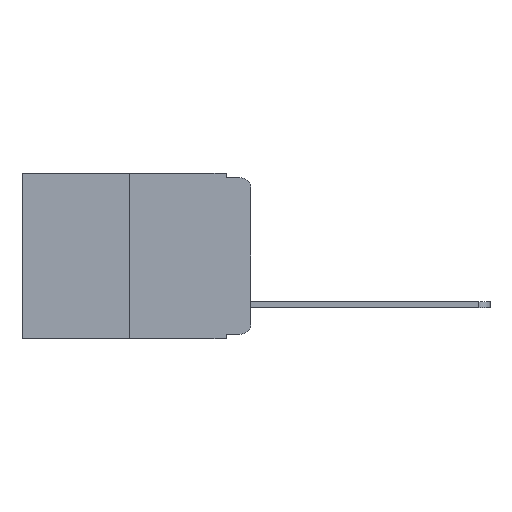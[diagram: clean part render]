
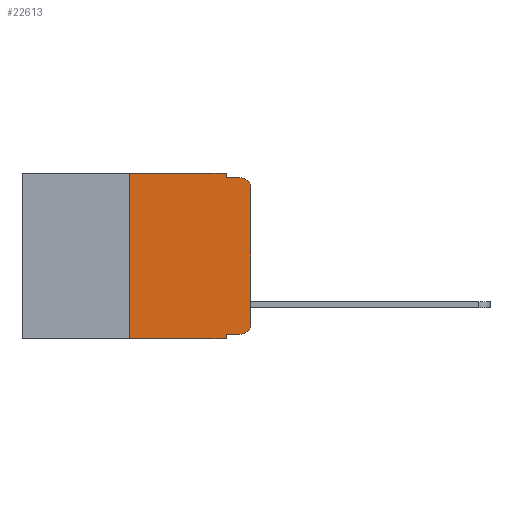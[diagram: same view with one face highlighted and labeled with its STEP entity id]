
A CAD part, left-side view. The second image highlights one B-rep face of the part: STEP entity #22613.
In plain terms, the highlighted planar face has unit normal (-1, 0, 0).
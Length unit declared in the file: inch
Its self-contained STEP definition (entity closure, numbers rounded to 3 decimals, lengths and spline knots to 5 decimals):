
#126 = DIRECTION ( 'NONE',  ( -1., 0., 0. ) ) ;
#195 = DIRECTION ( 'NONE',  ( 0., 0., -1. ) ) ;
#243 = DIRECTION ( 'NONE',  ( 0., 0., 1. ) ) ;
#452 = CARTESIAN_POINT ( 'NONE',  ( 0., 0., -0.03 ) ) ;
#665 = CARTESIAN_POINT ( 'NONE',  ( 0., 0.02, -0.03 ) ) ;
#1123 = DIRECTION ( 'NONE',  ( 0., -1., 0. ) ) ;
#1368 = EDGE_CURVE ( 'NONE', #11583, #18186, #4994, .T. ) ;
#1621 = VERTEX_POINT ( 'NONE', #452 ) ;
#1794 = CARTESIAN_POINT ( 'NONE',  ( 0., 0.02, -0.01 ) ) ;
#1830 = VECTOR ( 'NONE', #7894, 39.37008 ) ;
#2102 = LINE ( 'NONE', #6506, #6376 ) ;
#2175 = AXIS2_PLACEMENT_3D ( 'NONE', #3979, #126, #5667 ) ;
#2480 = AXIS2_PLACEMENT_3D ( 'NONE', #665, #10454, #17939 ) ;
#2651 = DIRECTION ( 'NONE',  ( 0., 0., 1. ) ) ;
#3492 = VERTEX_POINT ( 'NONE', #1794 ) ;
#3641 = ORIENTED_EDGE ( 'NONE', *, *, #16140, .F. ) ;
#3781 = LINE ( 'NONE', #5078, #24815 ) ;
#3979 = CARTESIAN_POINT ( 'NONE',  ( 0., 0.02, -0.313 ) ) ;
#4020 = DIRECTION ( 'NONE',  ( 0., 0., -1. ) ) ;
#4049 = VECTOR ( 'NONE', #11870, 39.37008 ) ;
#4238 = VERTEX_POINT ( 'NONE', #5587 ) ;
#4544 = VERTEX_POINT ( 'NONE', #23634 ) ;
#4590 = EDGE_CURVE ( 'NONE', #10619, #12416, #11844, .T. ) ;
#4672 = ORIENTED_EDGE ( 'NONE', *, *, #23143, .F. ) ;
#4930 = EDGE_CURVE ( 'NONE', #11583, #4544, #14873, .T. ) ;
#4994 = LINE ( 'NONE', #13523, #21528 ) ;
#5078 = CARTESIAN_POINT ( 'NONE',  ( 0., 0.051, -0.01 ) ) ;
#5170 = DIRECTION ( 'NONE',  ( 0., -1., 0. ) ) ;
#5285 = ORIENTED_EDGE ( 'NONE', *, *, #22074, .F. ) ;
#5587 = CARTESIAN_POINT ( 'NONE',  ( 0., 0.051, -0.01 ) ) ;
#5667 = DIRECTION ( 'NONE',  ( 0., 0., -1. ) ) ;
#5712 = CARTESIAN_POINT ( 'NONE',  ( 0., 0.051, 0. ) ) ;
#5719 = FACE_OUTER_BOUND ( 'NONE', #17930, .T. ) ;
#6213 = ORIENTED_EDGE ( 'NONE', *, *, #15669, .F. ) ;
#6376 = VECTOR ( 'NONE', #23713, 39.37008 ) ;
#6506 = CARTESIAN_POINT ( 'NONE',  ( 0., 0.051, 0. ) ) ;
#6698 = ORIENTED_EDGE ( 'NONE', *, *, #7846, .T. ) ;
#7539 = CIRCLE ( 'NONE', #2480, 0.02 ) ;
#7821 = EDGE_CURVE ( 'NONE', #1621, #3492, #7539, .T. ) ;
#7846 = EDGE_CURVE ( 'NONE', #10344, #1621, #19203, .T. ) ;
#7894 = DIRECTION ( 'NONE',  ( 0., -1., 0. ) ) ;
#8341 = EDGE_CURVE ( 'NONE', #12416, #10344, #22831, .T. ) ;
#9517 = VECTOR ( 'NONE', #1123, 39.37008 ) ;
#10344 = VERTEX_POINT ( 'NONE', #10960 ) ;
#10454 = DIRECTION ( 'NONE',  ( -1., 0., 0. ) ) ;
#10550 = ORIENTED_EDGE ( 'NONE', *, *, #8341, .T. ) ;
#10619 = VERTEX_POINT ( 'NONE', #17925 ) ;
#10960 = CARTESIAN_POINT ( 'NONE',  ( 0., 0., -0.313 ) ) ;
#11099 = ORIENTED_EDGE ( 'NONE', *, *, #4590, .T. ) ;
#11583 = VERTEX_POINT ( 'NONE', #16143 ) ;
#11828 = DIRECTION ( 'NONE',  ( 1., 0., 0. ) ) ;
#11844 = LINE ( 'NONE', #18854, #1830 ) ;
#11870 = DIRECTION ( 'NONE',  ( 0., -1., 0. ) ) ;
#12416 = VERTEX_POINT ( 'NONE', #15258 ) ;
#12830 = CARTESIAN_POINT ( 'NONE',  ( 0., 0.473, 0. ) ) ;
#13285 = VERTEX_POINT ( 'NONE', #18645 ) ;
#13523 = CARTESIAN_POINT ( 'NONE',  ( 0., 0.25, 0. ) ) ;
#14090 = CARTESIAN_POINT ( 'NONE',  ( 0., 0.25, 0. ) ) ;
#14173 = CARTESIAN_POINT ( 'NONE',  ( 0., 0., 0. ) ) ;
#14778 = ORIENTED_EDGE ( 'NONE', *, *, #7821, .T. ) ;
#14873 = LINE ( 'NONE', #19754, #4049 ) ;
#15258 = CARTESIAN_POINT ( 'NONE',  ( 0., 0.02, -0.333 ) ) ;
#15669 = EDGE_CURVE ( 'NONE', #4238, #3492, #3781, .T. ) ;
#15923 = VECTOR ( 'NONE', #2651, 39.37008 ) ;
#16140 = EDGE_CURVE ( 'NONE', #18186, #13285, #24200, .T. ) ;
#16143 = CARTESIAN_POINT ( 'NONE',  ( 0., 0.25, -0.343 ) ) ;
#16755 = AXIS2_PLACEMENT_3D ( 'NONE', #23288, #11828, #195 ) ;
#17378 = LINE ( 'NONE', #5712, #20997 ) ;
#17925 = CARTESIAN_POINT ( 'NONE',  ( 0., 0.051, -0.333 ) ) ;
#17930 = EDGE_LOOP ( 'NONE', ( #6698, #14778, #6213, #5285, #3641, #20723, #22760, #4672, #11099, #10550 ) ) ;
#17939 = DIRECTION ( 'NONE',  ( 0., 0., -1. ) ) ;
#18186 = VERTEX_POINT ( 'NONE', #14090 ) ;
#18645 = CARTESIAN_POINT ( 'NONE',  ( 0., 0.051, 0. ) ) ;
#18854 = CARTESIAN_POINT ( 'NONE',  ( 0., 0.051, -0.333 ) ) ;
#19203 = LINE ( 'NONE', #14173, #15923 ) ;
#19754 = CARTESIAN_POINT ( 'NONE',  ( 0., 0.473, -0.343 ) ) ;
#20723 = ORIENTED_EDGE ( 'NONE', *, *, #1368, .F. ) ;
#20997 = VECTOR ( 'NONE', #4020, 39.37008 ) ;
#21528 = VECTOR ( 'NONE', #243, 39.37008 ) ;
#22074 = EDGE_CURVE ( 'NONE', #13285, #4238, #2102, .T. ) ;
#22613 = ADVANCED_FACE ( 'NONE', ( #5719 ), #23530, .F. ) ;
#22760 = ORIENTED_EDGE ( 'NONE', *, *, #4930, .T. ) ;
#22831 = CIRCLE ( 'NONE', #2175, 0.02 ) ;
#23143 = EDGE_CURVE ( 'NONE', #10619, #4544, #17378, .T. ) ;
#23288 = CARTESIAN_POINT ( 'NONE',  ( 0., 0.473, 0. ) ) ;
#23530 = PLANE ( 'NONE',  #16755 ) ;
#23634 = CARTESIAN_POINT ( 'NONE',  ( 0., 0.051, -0.343 ) ) ;
#23713 = DIRECTION ( 'NONE',  ( 0., 0., -1. ) ) ;
#24200 = LINE ( 'NONE', #12830, #9517 ) ;
#24815 = VECTOR ( 'NONE', #5170, 39.37008 ) ;
